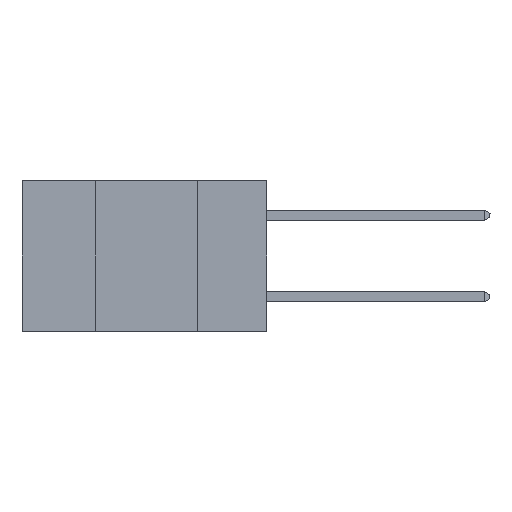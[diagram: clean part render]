
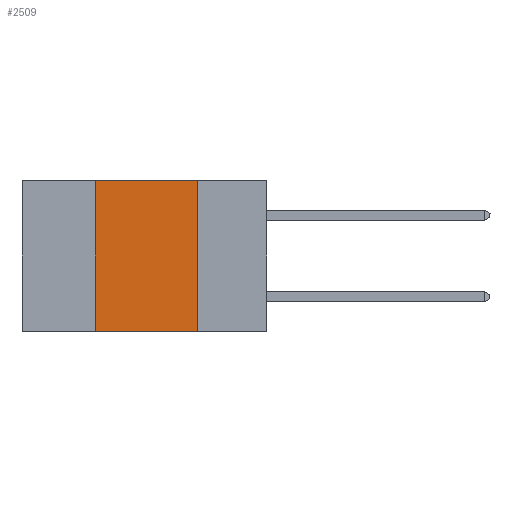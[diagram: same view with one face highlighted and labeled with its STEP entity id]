
A CAD part, left-side view. The second image highlights one B-rep face of the part: STEP entity #2509.
In plain terms, the highlighted planar face has unit normal (-1, 0, 0).
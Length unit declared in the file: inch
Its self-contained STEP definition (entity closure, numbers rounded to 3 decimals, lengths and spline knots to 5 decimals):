
#99 = EDGE_CURVE ( 'NONE', #11378, #9291, #4881, .T. ) ;
#171 = PLANE ( 'NONE',  #3794 ) ;
#518 = FACE_OUTER_BOUND ( 'NONE', #7206, .T. ) ;
#794 = ORIENTED_EDGE ( 'NONE', *, *, #99, .T. ) ;
#961 = CARTESIAN_POINT ( 'NONE',  ( 0., 0.6, 0. ) ) ;
#965 = CARTESIAN_POINT ( 'NONE',  ( 0., 0.6, 0. ) ) ;
#1875 = VECTOR ( 'NONE', #2103, 39.37008 ) ;
#1941 = VECTOR ( 'NONE', #8727, 39.37008 ) ;
#2103 = DIRECTION ( 'NONE',  ( 0., -1., 0. ) ) ;
#2509 = ADVANCED_FACE ( 'NONE', ( #518 ), #171, .F. ) ;
#3259 = VECTOR ( 'NONE', #6611, 39.37008 ) ;
#3333 = CARTESIAN_POINT ( 'NONE',  ( 0., 0.42, -0.37 ) ) ;
#3414 = DIRECTION ( 'NONE',  ( 1., 0., 0. ) ) ;
#3794 = AXIS2_PLACEMENT_3D ( 'NONE', #965, #3414, #4811 ) ;
#4501 = CARTESIAN_POINT ( 'NONE',  ( 0., 0.17, -0.37 ) ) ;
#4564 = VECTOR ( 'NONE', #10110, 39.37008 ) ;
#4811 = DIRECTION ( 'NONE',  ( 0., 0., -1. ) ) ;
#4881 = LINE ( 'NONE', #5926, #4564 ) ;
#5140 = ORIENTED_EDGE ( 'NONE', *, *, #11632, .F. ) ;
#5492 = ORIENTED_EDGE ( 'NONE', *, *, #7348, .F. ) ;
#5926 = CARTESIAN_POINT ( 'NONE',  ( 0., 0.6, -0.37 ) ) ;
#6575 = CARTESIAN_POINT ( 'NONE',  ( 0., 0.42, 0. ) ) ;
#6611 = DIRECTION ( 'NONE',  ( 0., 0., 1. ) ) ;
#7206 = EDGE_LOOP ( 'NONE', ( #5492, #12322, #5140, #794 ) ) ;
#7348 = EDGE_CURVE ( 'NONE', #10057, #9291, #9355, .T. ) ;
#7830 = CARTESIAN_POINT ( 'NONE',  ( 0., 0.17, 0. ) ) ;
#8539 = VERTEX_POINT ( 'NONE', #10866 ) ;
#8727 = DIRECTION ( 'NONE',  ( 0., 0., -1. ) ) ;
#9291 = VERTEX_POINT ( 'NONE', #4501 ) ;
#9355 = LINE ( 'NONE', #7830, #1941 ) ;
#10057 = VERTEX_POINT ( 'NONE', #11058 ) ;
#10110 = DIRECTION ( 'NONE',  ( 0., -1., 0. ) ) ;
#10866 = CARTESIAN_POINT ( 'NONE',  ( 0., 0.42, 0. ) ) ;
#10898 = LINE ( 'NONE', #6575, #3259 ) ;
#11058 = CARTESIAN_POINT ( 'NONE',  ( 0., 0.17, 0. ) ) ;
#11378 = VERTEX_POINT ( 'NONE', #3333 ) ;
#11632 = EDGE_CURVE ( 'NONE', #11378, #8539, #10898, .T. ) ;
#11855 = LINE ( 'NONE', #961, #1875 ) ;
#12050 = EDGE_CURVE ( 'NONE', #8539, #10057, #11855, .T. ) ;
#12322 = ORIENTED_EDGE ( 'NONE', *, *, #12050, .F. ) ;
